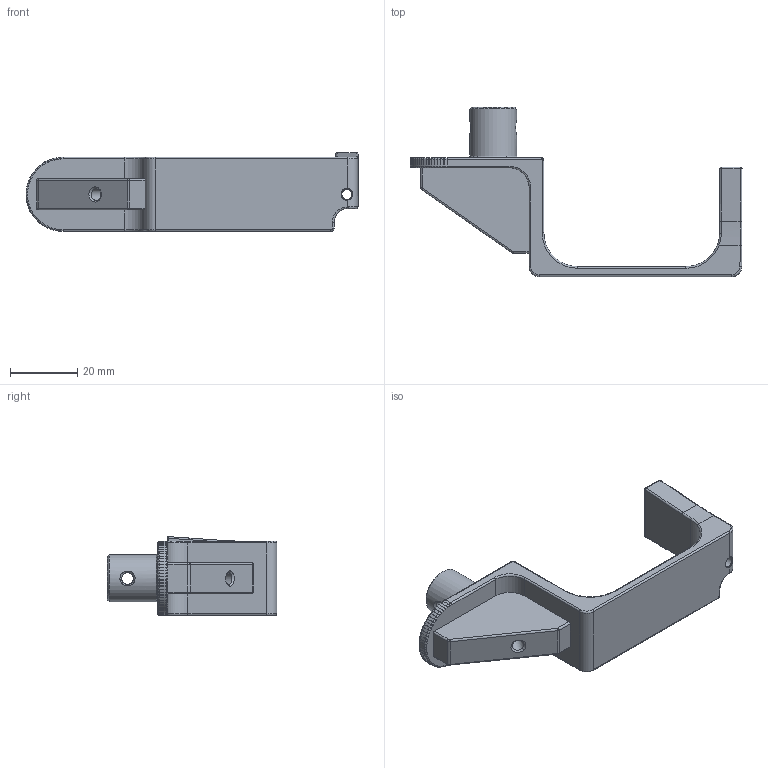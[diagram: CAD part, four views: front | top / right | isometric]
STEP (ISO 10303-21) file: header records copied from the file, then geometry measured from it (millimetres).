
FILE_DESCRIPTION(/* description */ (''),/* implementation_level */ '2;1');
FILE_NAME(/* name */ 'd27e20c4-aa20-4d49-aee9-35e1c3f8c06e.stp',/* time_stamp */ '2019-03-05T10:28:20-05:00',/* author */ ('suzuki450ltr'),/* organization */ (''),/* preprocessor_version */ 'ST-DEVELOPER v17.2',/* originating_system */ 'Autodesk Translation Framework v7.6.0.251',/* authorisation */ '');
FILE_SCHEMA (('AUTOMOTIVE_DESIGN { 1 0 10303 214 3 1 1 }'));
Length unit declared in the file: millimetre
Products named in the file (1): Vz61 Ar15 Grip Adapter Prototype v5_Vz61 Ar15 Grip Adapter Prototype 
v5
Bounding box: 98.83 x 50.4 x 23.47 mm (x, y, z)
Volume: 20422.7 mm3; surface area: 9915.3 mm2
Topology: 1 solids, 1 shells, 339 faces, 792 edges, 452 vertices
Faces by surface type: cylinder 159, bspline 93, plane 59, torus 14, sphere 10, cone 4
Full cylindrical faces by diameter (mm): 3 x1, 3.5 x1, 14.049 x1
Entity records: 10837 total; most frequent: CARTESIAN_POINT 3226, DIRECTION 1678, ORIENTED_EDGE 1578, EDGE_CURVE 789, AXIS2_PLACEMENT_3D 671, VERTEX_POINT 452, CIRCLE 424, EDGE_LOOP 343
